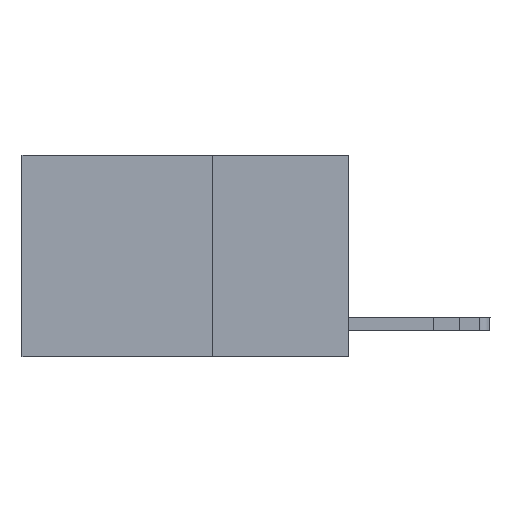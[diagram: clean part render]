
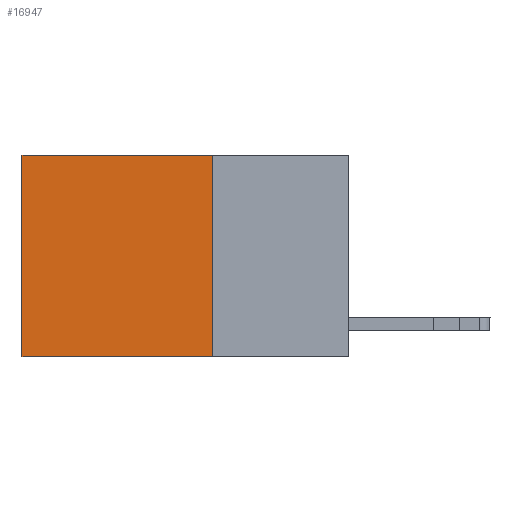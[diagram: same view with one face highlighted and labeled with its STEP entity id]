
A CAD part, left-side view. The second image highlights one B-rep face of the part: STEP entity #16947.
In plain terms, the highlighted planar face has unit normal (-1, 0, 0).
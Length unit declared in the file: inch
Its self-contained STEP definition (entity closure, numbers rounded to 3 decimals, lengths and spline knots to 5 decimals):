
#51 = LINE ( 'NONE', #7232, #6447 ) ;
#271 = VECTOR ( 'NONE', #14522, 39.37008 ) ;
#336 = LINE ( 'NONE', #5819, #271 ) ;
#402 = LINE ( 'NONE', #6453, #4679 ) ;
#1840 = ORIENTED_EDGE ( 'NONE', *, *, #2170, .F. ) ;
#1973 = VERTEX_POINT ( 'NONE', #18192 ) ;
#2018 = CARTESIAN_POINT ( 'NONE',  ( 0.2625, 0.6, 0. ) ) ;
#2170 = EDGE_CURVE ( 'NONE', #17446, #8776, #51, .T. ) ;
#4199 = EDGE_LOOP ( 'NONE', ( #10691, #15876, #1840, #15664 ) ) ;
#4562 = DIRECTION ( 'NONE',  ( 0., 0., -1. ) ) ;
#4679 = VECTOR ( 'NONE', #7867, 39.37008 ) ;
#4776 = EDGE_CURVE ( 'NONE', #17446, #15587, #402, .T. ) ;
#5819 = CARTESIAN_POINT ( 'NONE',  ( 0.2625, 0.6, 0. ) ) ;
#5968 = PLANE ( 'NONE',  #7566 ) ;
#6447 = VECTOR ( 'NONE', #18650, 39.37008 ) ;
#6453 = CARTESIAN_POINT ( 'NONE',  ( 0.2625, 0.25, 0. ) ) ;
#6678 = CARTESIAN_POINT ( 'NONE',  ( 0.2625, 0.25, -0.37 ) ) ;
#7232 = CARTESIAN_POINT ( 'NONE',  ( 0.2625, 0.25, 0. ) ) ;
#7566 = AXIS2_PLACEMENT_3D ( 'NONE', #11739, #17402, #4562 ) ;
#7867 = DIRECTION ( 'NONE',  ( 0., 1., 0. ) ) ;
#8776 = VERTEX_POINT ( 'NONE', #6678 ) ;
#10095 = EDGE_CURVE ( 'NONE', #8776, #1973, #12287, .T. ) ;
#10691 = ORIENTED_EDGE ( 'NONE', *, *, #12580, .T. ) ;
#11134 = VECTOR ( 'NONE', #16616, 39.37008 ) ;
#11645 = FACE_OUTER_BOUND ( 'NONE', #4199, .T. ) ;
#11739 = CARTESIAN_POINT ( 'NONE',  ( 0.2625, 0.25, 0. ) ) ;
#12287 = LINE ( 'NONE', #18021, #11134 ) ;
#12580 = EDGE_CURVE ( 'NONE', #15587, #1973, #336, .T. ) ;
#13614 = CARTESIAN_POINT ( 'NONE',  ( 0.2625, 0.25, 0. ) ) ;
#14522 = DIRECTION ( 'NONE',  ( 0., 0., -1. ) ) ;
#15587 = VERTEX_POINT ( 'NONE', #2018 ) ;
#15664 = ORIENTED_EDGE ( 'NONE', *, *, #4776, .T. ) ;
#15876 = ORIENTED_EDGE ( 'NONE', *, *, #10095, .F. ) ;
#16616 = DIRECTION ( 'NONE',  ( 0., 1., 0. ) ) ;
#16947 = ADVANCED_FACE ( 'NONE', ( #11645 ), #5968, .F. ) ;
#17402 = DIRECTION ( 'NONE',  ( 1., 0., 0. ) ) ;
#17446 = VERTEX_POINT ( 'NONE', #13614 ) ;
#18021 = CARTESIAN_POINT ( 'NONE',  ( 0.2625, 0.25, -0.37 ) ) ;
#18192 = CARTESIAN_POINT ( 'NONE',  ( 0.2625, 0.6, -0.37 ) ) ;
#18650 = DIRECTION ( 'NONE',  ( 0., 0., -1. ) ) ;
